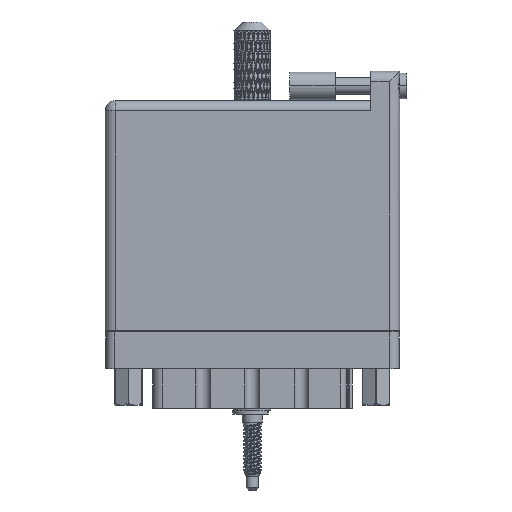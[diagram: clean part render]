
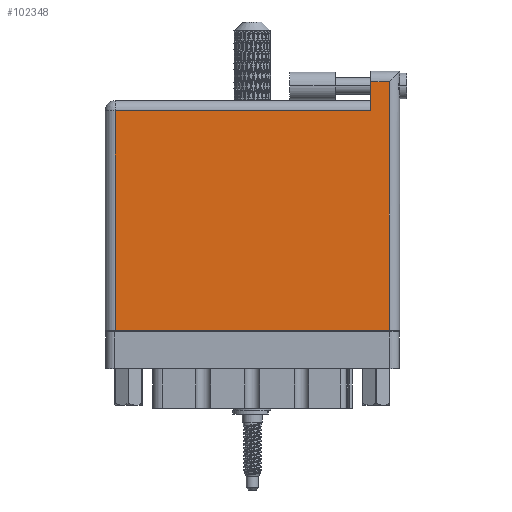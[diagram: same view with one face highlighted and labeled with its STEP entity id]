
A CAD part, front view. The second image highlights one B-rep face of the part: STEP entity #102348.
In plain terms, the highlighted face is planar.
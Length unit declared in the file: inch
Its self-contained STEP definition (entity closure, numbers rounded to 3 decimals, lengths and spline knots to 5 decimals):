
#1935 = DIRECTION ( 'NONE',  ( -1., 0., 0. ) ) ;
#3022 = VECTOR ( 'NONE', #74271, 39.37008 ) ;
#6910 = VECTOR ( 'NONE', #23309, 39.37008 ) ;
#8693 = VERTEX_POINT ( 'NONE', #36658 ) ;
#8841 = FACE_OUTER_BOUND ( 'NONE', #71473, .T. ) ;
#9633 = LINE ( 'NONE', #75406, #52844 ) ;
#11857 = CARTESIAN_POINT ( 'NONE',  ( 0., 0., 0. ) ) ;
#11921 = CARTESIAN_POINT ( 'NONE',  ( 0.07, 0., 0. ) ) ;
#20720 = PLANE ( 'NONE',  #97850 ) ;
#21721 = VERTEX_POINT ( 'NONE', #104889 ) ;
#22238 = ORIENTED_EDGE ( 'NONE', *, *, #62714, .T. ) ;
#23309 = DIRECTION ( 'NONE',  ( 0., 1., 0. ) ) ;
#24904 = EDGE_CURVE ( 'NONE', #35867, #36894, #9633, .T. ) ;
#31052 = DIRECTION ( 'NONE',  ( 0., -1., 0. ) ) ;
#31542 = CARTESIAN_POINT ( 'NONE',  ( 1.938, 1.696, 0. ) ) ;
#35867 = VERTEX_POINT ( 'NONE', #105525 ) ;
#36658 = CARTESIAN_POINT ( 'NONE',  ( 0.07, 1.496, 0. ) ) ;
#36894 = VERTEX_POINT ( 'NONE', #97043 ) ;
#37367 = LINE ( 'NONE', #93285, #41500 ) ;
#37379 = CARTESIAN_POINT ( 'NONE',  ( 0., 1.696, 0. ) ) ;
#37870 = ORIENTED_EDGE ( 'NONE', *, *, #74889, .T. ) ;
#39383 = VERTEX_POINT ( 'NONE', #31542 ) ;
#41500 = VECTOR ( 'NONE', #48885, 39.37008 ) ;
#45191 = ORIENTED_EDGE ( 'NONE', *, *, #45883, .T. ) ;
#45883 = EDGE_CURVE ( 'NONE', #8693, #81852, #100545, .T. ) ;
#48006 = DIRECTION ( 'NONE',  ( -1., 0., 0. ) ) ;
#48885 = DIRECTION ( 'NONE',  ( -1., 0., 0. ) ) ;
#50208 = CARTESIAN_POINT ( 'NONE',  ( 1.938, 1.766, 0. ) ) ;
#52844 = VECTOR ( 'NONE', #31052, 39.37008 ) ;
#56229 = CARTESIAN_POINT ( 'NONE',  ( 0., 1.566, 0. ) ) ;
#56672 = LINE ( 'NONE', #11857, #67829 ) ;
#56676 = EDGE_CURVE ( 'NONE', #81852, #21721, #56672, .T. ) ;
#57481 = CARTESIAN_POINT ( 'NONE',  ( 0.07, 0., 0. ) ) ;
#59186 = ORIENTED_EDGE ( 'NONE', *, *, #56676, .T. ) ;
#59872 = LINE ( 'NONE', #50208, #6910 ) ;
#62714 = EDGE_CURVE ( 'NONE', #36894, #8693, #37367, .T. ) ;
#65103 = VECTOR ( 'NONE', #1935, 39.37008 ) ;
#67829 = VECTOR ( 'NONE', #70279, 39.37008 ) ;
#70279 = DIRECTION ( 'NONE',  ( 1., 0., 0. ) ) ;
#71473 = EDGE_LOOP ( 'NONE', ( #59186, #108539, #37870, #113726, #22238, #45191 ) ) ;
#74271 = DIRECTION ( 'NONE',  ( 0., -1., 0. ) ) ;
#74889 = EDGE_CURVE ( 'NONE', #39383, #35867, #91619, .T. ) ;
#75406 = CARTESIAN_POINT ( 'NONE',  ( 1.811, 1.766, 0. ) ) ;
#81852 = VERTEX_POINT ( 'NONE', #57481 ) ;
#83033 = DIRECTION ( 'NONE',  ( 0., 0., -1. ) ) ;
#91619 = LINE ( 'NONE', #37379, #65103 ) ;
#93285 = CARTESIAN_POINT ( 'NONE',  ( 0., 1.496, 0. ) ) ;
#97043 = CARTESIAN_POINT ( 'NONE',  ( 1.811, 1.496, 0. ) ) ;
#97850 = AXIS2_PLACEMENT_3D ( 'NONE', #56229, #83033, #48006 ) ;
#100545 = LINE ( 'NONE', #11921, #3022 ) ;
#101632 = EDGE_CURVE ( 'NONE', #21721, #39383, #59872, .T. ) ;
#102348 = ADVANCED_FACE ( 'NONE', ( #8841 ), #20720, .F. ) ;
#104889 = CARTESIAN_POINT ( 'NONE',  ( 1.938, 0., 0. ) ) ;
#105525 = CARTESIAN_POINT ( 'NONE',  ( 1.811, 1.696, 0. ) ) ;
#108539 = ORIENTED_EDGE ( 'NONE', *, *, #101632, .T. ) ;
#113726 = ORIENTED_EDGE ( 'NONE', *, *, #24904, .T. ) ;
